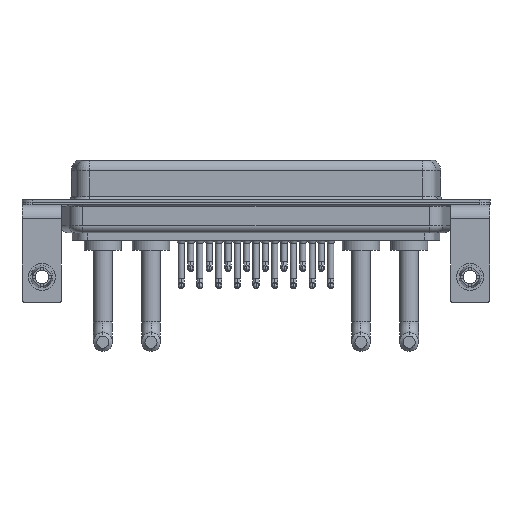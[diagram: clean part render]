
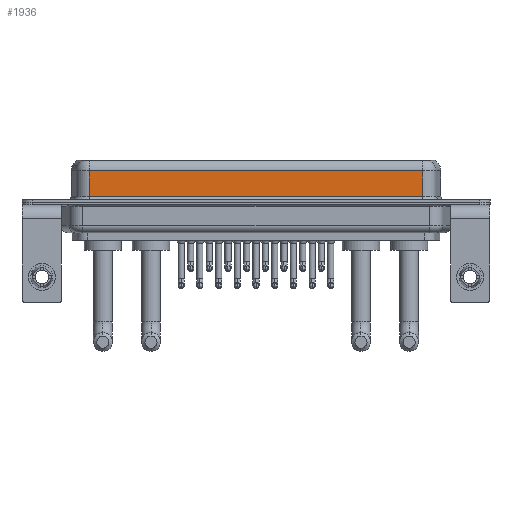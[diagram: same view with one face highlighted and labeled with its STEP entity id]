
A CAD part, front view. The second image highlights one B-rep face of the part: STEP entity #1936.
In plain terms, the highlighted planar face has unit normal (0, -1, 0).
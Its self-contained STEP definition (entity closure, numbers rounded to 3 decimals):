
#552 = FACE_OUTER_BOUND ( 'NONE', #11247, .T. ) ;
#838 = ORIENTED_EDGE ( 'NONE', *, *, #3867, .T. ) ;
#1050 = VERTEX_POINT ( 'NONE', #11893 ) ;
#1074 = VECTOR ( 'NONE', #9839, 1000. ) ;
#1281 = VERTEX_POINT ( 'NONE', #12495 ) ;
#1936 = ADVANCED_FACE ( 'NONE', ( #552 ), #7969, .F. ) ;
#2292 = CARTESIAN_POINT ( 'NONE',  ( 7.038, -3.95, 6.4 ) ) ;
#3867 = EDGE_CURVE ( 'NONE', #23440, #1281, #6955, .T. ) ;
#4515 = CARTESIAN_POINT ( 'NONE',  ( 56.462, -3.95, 6.4 ) ) ;
#6400 = EDGE_CURVE ( 'NONE', #1050, #21613, #10113, .T. ) ;
#6955 = LINE ( 'NONE', #21916, #16256 ) ;
#7745 = CARTESIAN_POINT ( 'NONE',  ( 56.462, -3.95, 6.4 ) ) ;
#7969 = PLANE ( 'NONE',  #9396 ) ;
#8085 = DIRECTION ( 'NONE',  ( 0., 1., 0. ) ) ;
#8510 = DIRECTION ( 'NONE',  ( 1., 0., 0. ) ) ;
#8716 = ORIENTED_EDGE ( 'NONE', *, *, #18733, .F. ) ;
#8933 = DIRECTION ( 'NONE',  ( -1., 0., 0. ) ) ;
#9396 = AXIS2_PLACEMENT_3D ( 'NONE', #4515, #8085, #17604 ) ;
#9839 = DIRECTION ( 'NONE',  ( 0., 0., -1. ) ) ;
#10113 = LINE ( 'NONE', #17657, #17668 ) ;
#11115 = CARTESIAN_POINT ( 'NONE',  ( 56.462, -3.95, 0.9 ) ) ;
#11247 = EDGE_LOOP ( 'NONE', ( #8716, #838, #20197, #14065 ) ) ;
#11893 = CARTESIAN_POINT ( 'NONE',  ( 7.038, -3.95, 0.9 ) ) ;
#12495 = CARTESIAN_POINT ( 'NONE',  ( 7.038, -3.95, 4.65 ) ) ;
#13306 = LINE ( 'NONE', #7745, #16721 ) ;
#14065 = ORIENTED_EDGE ( 'NONE', *, *, #6400, .T. ) ;
#16256 = VECTOR ( 'NONE', #8933, 1000. ) ;
#16721 = VECTOR ( 'NONE', #20966, 1000. ) ;
#17604 = DIRECTION ( 'NONE',  ( 0., 0., 1. ) ) ;
#17657 = CARTESIAN_POINT ( 'NONE',  ( 56.462, -3.95, 0.9 ) ) ;
#17668 = VECTOR ( 'NONE', #8510, 1000. ) ;
#18733 = EDGE_CURVE ( 'NONE', #23440, #21613, #13306, .T. ) ;
#18839 = EDGE_CURVE ( 'NONE', #1281, #1050, #23051, .T. ) ;
#20197 = ORIENTED_EDGE ( 'NONE', *, *, #18839, .T. ) ;
#20966 = DIRECTION ( 'NONE',  ( 0., 0., -1. ) ) ;
#21613 = VERTEX_POINT ( 'NONE', #11115 ) ;
#21840 = CARTESIAN_POINT ( 'NONE',  ( 56.462, -3.95, 4.65 ) ) ;
#21916 = CARTESIAN_POINT ( 'NONE',  ( 56.462, -3.95, 4.65 ) ) ;
#23051 = LINE ( 'NONE', #2292, #1074 ) ;
#23440 = VERTEX_POINT ( 'NONE', #21840 ) ;
